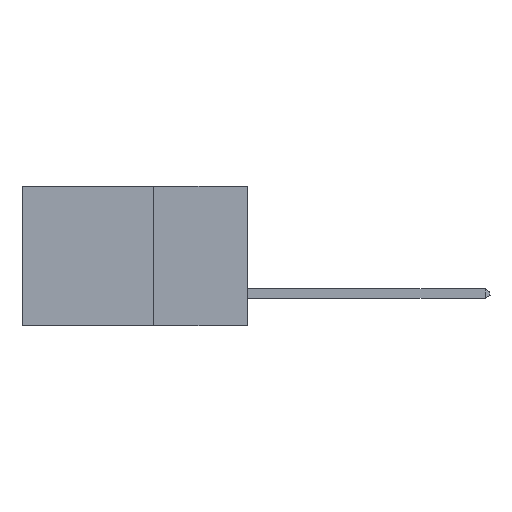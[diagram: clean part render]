
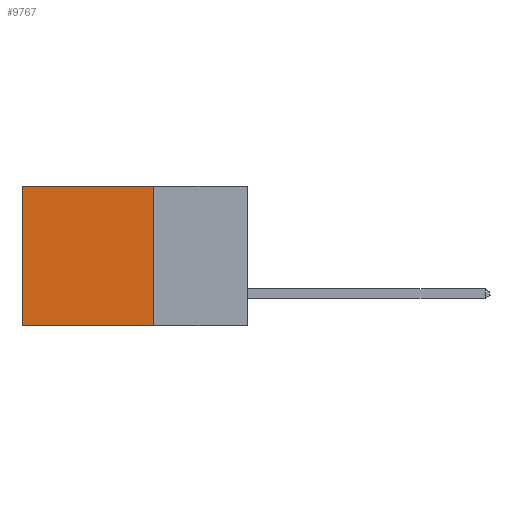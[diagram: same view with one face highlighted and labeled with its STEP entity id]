
A CAD part, left-side view. The second image highlights one B-rep face of the part: STEP entity #9767.
In plain terms, the highlighted planar face has unit normal (-1, 0, 0).
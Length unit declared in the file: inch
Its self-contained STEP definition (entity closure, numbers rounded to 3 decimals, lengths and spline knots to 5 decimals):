
#339 = EDGE_CURVE ( 'NONE', #17945, #6758, #3225, .T. ) ;
#553 = ORIENTED_EDGE ( 'NONE', *, *, #14642, .F. ) ;
#989 = LINE ( 'NONE', #17518, #8974 ) ;
#1046 = ORIENTED_EDGE ( 'NONE', *, *, #339, .F. ) ;
#1347 = EDGE_CURVE ( 'NONE', #17945, #10707, #5267, .T. ) ;
#1627 = LINE ( 'NONE', #19298, #14306 ) ;
#2695 = VECTOR ( 'NONE', #18386, 39.37008 ) ;
#3225 = LINE ( 'NONE', #5127, #2695 ) ;
#3964 = CARTESIAN_POINT ( 'NONE',  ( 0.298, 0.25, 0. ) ) ;
#4105 = DIRECTION ( 'NONE',  ( 0., 1., 0. ) ) ;
#4474 = VERTEX_POINT ( 'NONE', #17319 ) ;
#4752 = VECTOR ( 'NONE', #4105, 39.37008 ) ;
#5127 = CARTESIAN_POINT ( 'NONE',  ( 0.298, 0.25, 0. ) ) ;
#5267 = LINE ( 'NONE', #5690, #4752 ) ;
#5674 = PLANE ( 'NONE',  #13175 ) ;
#5690 = CARTESIAN_POINT ( 'NONE',  ( 0.298, 0.25, 0. ) ) ;
#6562 = CARTESIAN_POINT ( 'NONE',  ( 0.298, 0.25, -0.37 ) ) ;
#6758 = VERTEX_POINT ( 'NONE', #6562 ) ;
#7195 = CARTESIAN_POINT ( 'NONE',  ( 0.298, 0.25, 0. ) ) ;
#7290 = DIRECTION ( 'NONE',  ( 0., 0., -1. ) ) ;
#7681 = DIRECTION ( 'NONE',  ( 0., 0., -1. ) ) ;
#8196 = EDGE_LOOP ( 'NONE', ( #8270, #553, #1046, #14769 ) ) ;
#8270 = ORIENTED_EDGE ( 'NONE', *, *, #18820, .T. ) ;
#8974 = VECTOR ( 'NONE', #7681, 39.37008 ) ;
#9767 = ADVANCED_FACE ( 'NONE', ( #15169 ), #5674, .F. ) ;
#10707 = VERTEX_POINT ( 'NONE', #15047 ) ;
#13175 = AXIS2_PLACEMENT_3D ( 'NONE', #3964, #20605, #7290 ) ;
#14306 = VECTOR ( 'NONE', #20928, 39.37008 ) ;
#14642 = EDGE_CURVE ( 'NONE', #6758, #4474, #1627, .T. ) ;
#14769 = ORIENTED_EDGE ( 'NONE', *, *, #1347, .T. ) ;
#15047 = CARTESIAN_POINT ( 'NONE',  ( 0.298, 0.6, 0. ) ) ;
#15169 = FACE_OUTER_BOUND ( 'NONE', #8196, .T. ) ;
#17319 = CARTESIAN_POINT ( 'NONE',  ( 0.298, 0.6, -0.37 ) ) ;
#17518 = CARTESIAN_POINT ( 'NONE',  ( 0.298, 0.6, 0. ) ) ;
#17945 = VERTEX_POINT ( 'NONE', #7195 ) ;
#18386 = DIRECTION ( 'NONE',  ( 0., 0., -1. ) ) ;
#18820 = EDGE_CURVE ( 'NONE', #10707, #4474, #989, .T. ) ;
#19298 = CARTESIAN_POINT ( 'NONE',  ( 0.298, 0.25, -0.37 ) ) ;
#20605 = DIRECTION ( 'NONE',  ( 1., 0., 0. ) ) ;
#20928 = DIRECTION ( 'NONE',  ( 0., 1., 0. ) ) ;
